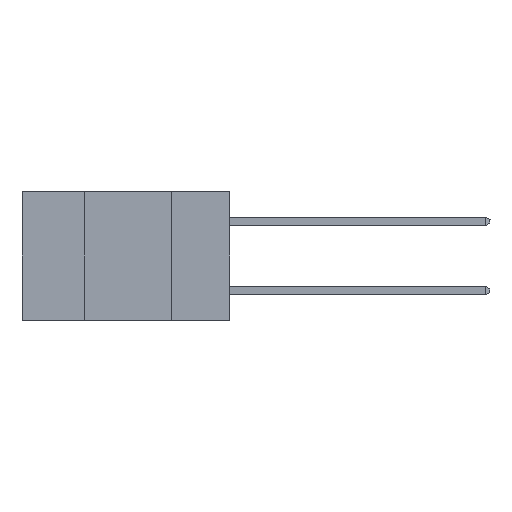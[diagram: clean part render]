
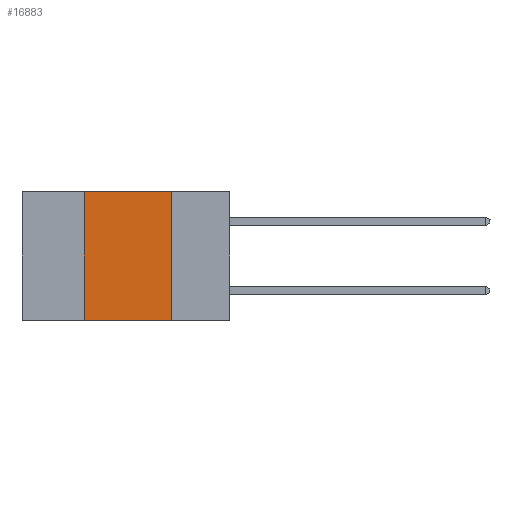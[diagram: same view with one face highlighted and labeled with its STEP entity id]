
A CAD part, left-side view. The second image highlights one B-rep face of the part: STEP entity #16883.
In plain terms, the highlighted planar face has unit normal (-1, 0, 0).
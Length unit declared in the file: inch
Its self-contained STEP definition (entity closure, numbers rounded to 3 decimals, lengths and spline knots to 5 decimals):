
#1601 = VECTOR ( 'NONE', #20875, 39.37008 ) ;
#2380 = LINE ( 'NONE', #9638, #10727 ) ;
#3227 = CARTESIAN_POINT ( 'NONE',  ( 0., 0.42, -0.37 ) ) ;
#4409 = DIRECTION ( 'NONE',  ( 1., 0., 0. ) ) ;
#6684 = VERTEX_POINT ( 'NONE', #12240 ) ;
#7824 = CARTESIAN_POINT ( 'NONE',  ( 0., 0.17, -0.37 ) ) ;
#7973 = FACE_OUTER_BOUND ( 'NONE', #13677, .T. ) ;
#8445 = VERTEX_POINT ( 'NONE', #21133 ) ;
#8638 = EDGE_CURVE ( 'NONE', #10741, #16139, #17077, .T. ) ;
#9594 = ORIENTED_EDGE ( 'NONE', *, *, #13378, .F. ) ;
#9638 = CARTESIAN_POINT ( 'NONE',  ( 0., 0.6, -0.37 ) ) ;
#10417 = PLANE ( 'NONE',  #16554 ) ;
#10727 = VECTOR ( 'NONE', #16362, 39.37008 ) ;
#10741 = VERTEX_POINT ( 'NONE', #20071 ) ;
#11871 = DIRECTION ( 'NONE',  ( 0., 0., -1. ) ) ;
#12240 = CARTESIAN_POINT ( 'NONE',  ( 0., 0.42, -0.37 ) ) ;
#13205 = DIRECTION ( 'NONE',  ( 0., -1., 0. ) ) ;
#13376 = VECTOR ( 'NONE', #18378, 39.37008 ) ;
#13378 = EDGE_CURVE ( 'NONE', #6684, #8445, #23882, .T. ) ;
#13677 = EDGE_LOOP ( 'NONE', ( #16851, #20655, #9594, #20484 ) ) ;
#13810 = CARTESIAN_POINT ( 'NONE',  ( 0., 0.6, 0. ) ) ;
#16139 = VERTEX_POINT ( 'NONE', #20000 ) ;
#16362 = DIRECTION ( 'NONE',  ( 0., -1., 0. ) ) ;
#16554 = AXIS2_PLACEMENT_3D ( 'NONE', #13810, #4409, #11871 ) ;
#16851 = ORIENTED_EDGE ( 'NONE', *, *, #8638, .F. ) ;
#16883 = ADVANCED_FACE ( 'NONE', ( #7973 ), #10417, .F. ) ;
#17077 = LINE ( 'NONE', #7824, #1601 ) ;
#18378 = DIRECTION ( 'NONE',  ( 0., 0., 1. ) ) ;
#19286 = EDGE_CURVE ( 'NONE', #8445, #10741, #20890, .T. ) ;
#20000 = CARTESIAN_POINT ( 'NONE',  ( 0., 0.17, -0.37 ) ) ;
#20071 = CARTESIAN_POINT ( 'NONE',  ( 0., 0.17, 0. ) ) ;
#20484 = ORIENTED_EDGE ( 'NONE', *, *, #23444, .T. ) ;
#20655 = ORIENTED_EDGE ( 'NONE', *, *, #19286, .F. ) ;
#20875 = DIRECTION ( 'NONE',  ( 0., 0., -1. ) ) ;
#20890 = LINE ( 'NONE', #22606, #24064 ) ;
#21133 = CARTESIAN_POINT ( 'NONE',  ( 0., 0.42, 0. ) ) ;
#22606 = CARTESIAN_POINT ( 'NONE',  ( 0., 0.6, 0. ) ) ;
#23444 = EDGE_CURVE ( 'NONE', #6684, #16139, #2380, .T. ) ;
#23882 = LINE ( 'NONE', #3227, #13376 ) ;
#24064 = VECTOR ( 'NONE', #13205, 39.37008 ) ;
